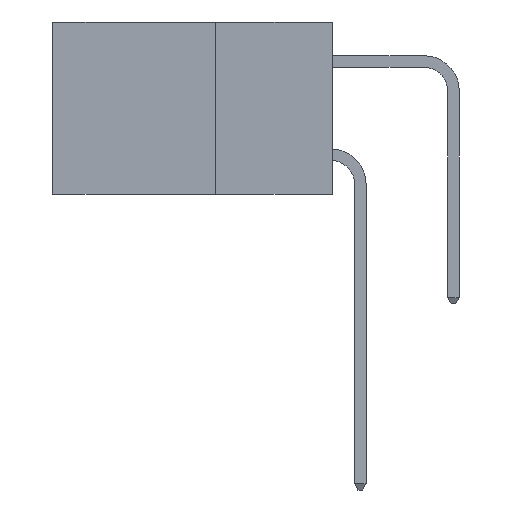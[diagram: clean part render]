
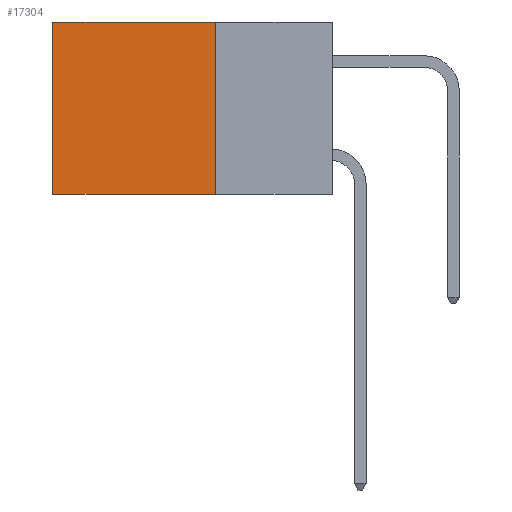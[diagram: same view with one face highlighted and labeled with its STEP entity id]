
A CAD part, left-side view. The second image highlights one B-rep face of the part: STEP entity #17304.
In plain terms, the highlighted planar face has unit normal (-1, 0, 0).
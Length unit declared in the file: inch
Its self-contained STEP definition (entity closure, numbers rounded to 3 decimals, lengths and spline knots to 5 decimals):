
#559 = ORIENTED_EDGE ( 'NONE', *, *, #11160, .F. ) ;
#1457 = DIRECTION ( 'NONE',  ( 1., 0., 0. ) ) ;
#2374 = LINE ( 'NONE', #8946, #16852 ) ;
#3516 = VERTEX_POINT ( 'NONE', #5507 ) ;
#4008 = EDGE_LOOP ( 'NONE', ( #15342, #4904, #559, #4709 ) ) ;
#4155 = CARTESIAN_POINT ( 'NONE',  ( 0.2615, 0.6, 0. ) ) ;
#4601 = CARTESIAN_POINT ( 'NONE',  ( 0.2615, 0.25, -0.37 ) ) ;
#4709 = ORIENTED_EDGE ( 'NONE', *, *, #14888, .T. ) ;
#4904 = ORIENTED_EDGE ( 'NONE', *, *, #16827, .F. ) ;
#5507 = CARTESIAN_POINT ( 'NONE',  ( 0.2615, 0.25, -0.37 ) ) ;
#6135 = LINE ( 'NONE', #4601, #10284 ) ;
#6913 = LINE ( 'NONE', #8318, #15039 ) ;
#6972 = PLANE ( 'NONE',  #9093 ) ;
#8318 = CARTESIAN_POINT ( 'NONE',  ( 0.2615, 0.6, -0.37 ) ) ;
#8838 = DIRECTION ( 'NONE',  ( 0., 1., 0. ) ) ;
#8941 = DIRECTION ( 'NONE',  ( 0., 0., -1. ) ) ;
#8946 = CARTESIAN_POINT ( 'NONE',  ( 0.2615, 0.25, -0.37 ) ) ;
#9093 = AXIS2_PLACEMENT_3D ( 'NONE', #9764, #1457, #11197 ) ;
#9764 = CARTESIAN_POINT ( 'NONE',  ( 0.2615, 0.25, -0.37 ) ) ;
#10275 = CARTESIAN_POINT ( 'NONE',  ( 0.2615, 0.25, 0. ) ) ;
#10284 = VECTOR ( 'NONE', #8838, 39.37008 ) ;
#11160 = EDGE_CURVE ( 'NONE', #13117, #3516, #2374, .T. ) ;
#11197 = DIRECTION ( 'NONE',  ( 0., 0., -1. ) ) ;
#11630 = VERTEX_POINT ( 'NONE', #4155 ) ;
#12202 = FACE_OUTER_BOUND ( 'NONE', #4008, .T. ) ;
#13117 = VERTEX_POINT ( 'NONE', #17494 ) ;
#13184 = EDGE_CURVE ( 'NONE', #11630, #13881, #6913, .T. ) ;
#13881 = VERTEX_POINT ( 'NONE', #15135 ) ;
#14450 = DIRECTION ( 'NONE',  ( 0., 1., 0. ) ) ;
#14584 = VECTOR ( 'NONE', #14450, 39.37008 ) ;
#14888 = EDGE_CURVE ( 'NONE', #13117, #11630, #14973, .T. ) ;
#14973 = LINE ( 'NONE', #10275, #14584 ) ;
#15039 = VECTOR ( 'NONE', #16370, 39.37008 ) ;
#15135 = CARTESIAN_POINT ( 'NONE',  ( 0.2615, 0.6, -0.37 ) ) ;
#15342 = ORIENTED_EDGE ( 'NONE', *, *, #13184, .T. ) ;
#16370 = DIRECTION ( 'NONE',  ( 0., 0., -1. ) ) ;
#16827 = EDGE_CURVE ( 'NONE', #3516, #13881, #6135, .T. ) ;
#16852 = VECTOR ( 'NONE', #8941, 39.37008 ) ;
#17304 = ADVANCED_FACE ( 'NONE', ( #12202 ), #6972, .F. ) ;
#17494 = CARTESIAN_POINT ( 'NONE',  ( 0.2615, 0.25, 0. ) ) ;
